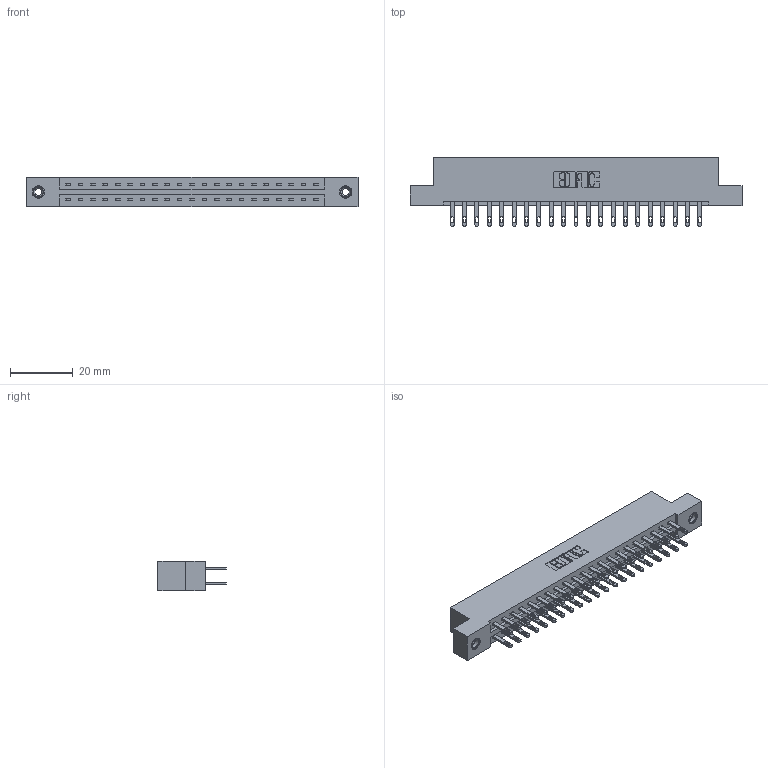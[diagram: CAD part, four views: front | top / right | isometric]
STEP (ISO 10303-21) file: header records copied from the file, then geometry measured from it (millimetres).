
FILE_DESCRIPTION (( 'STEP AP203' ), '1' );
FILE_NAME ('887-042-500-208.STEP', '2020-09-21T00:00:27', ( '' ), ( '' ), 'SwSTEP 2.0', 'SolidWorks 2020', '' );
FILE_SCHEMA (( 'CONFIG_CONTROL_DESIGN' ));
Length unit declared in the file: inch
Products named in the file (4): 345-292-001_345-293-100; 837 Part_Flush Mounting Lugs - 0.156 Dia-TI; 345-250-001_345-250-003-102; 887-042-500-208
Assembly tree (45 placements, depth 2):
  887-042-500-208
    837 Part_Flush Mounting Lugs - 0.156 Dia-TI
    345-292-001_345-293-100  x42
    345-250-001_345-250-003-102  x2
Bounding box: 106.22 x 21.85 x 9.4 mm (x, y, z)
Volume: 11036.9 mm3; surface area: 12763.2 mm2
Topology: 45 solids, 45 shells, 2274 faces, 6873 edges, 4574 vertices
Faces by surface type: plane 1446, cylinder 812, cone 12, torus 4
Entity records: 20114 total; most frequent: CARTESIAN_POINT 3385, ORIENTED_EDGE 3314, DIRECTION 2951, EDGE_CURVE 1657, VECTOR 1505, LINE 1505, VERTEX_POINT 1100, AXIS2_PLACEMENT_3D 723
